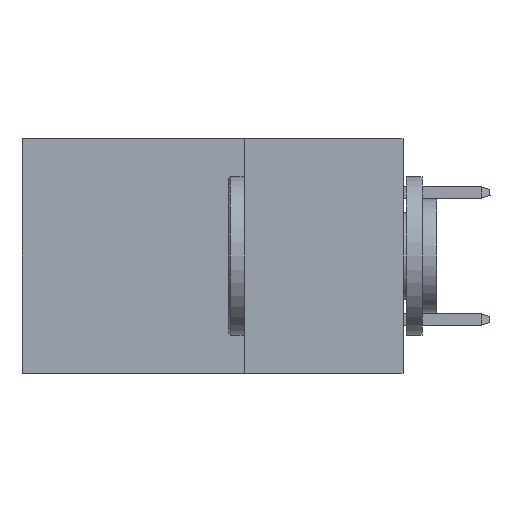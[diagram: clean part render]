
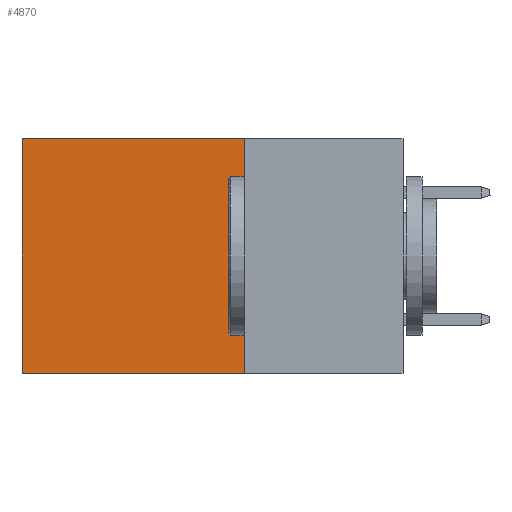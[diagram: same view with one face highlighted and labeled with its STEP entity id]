
A CAD part, left-side view. The second image highlights one B-rep face of the part: STEP entity #4870.
In plain terms, the highlighted planar face has unit normal (-1, 0, 0).
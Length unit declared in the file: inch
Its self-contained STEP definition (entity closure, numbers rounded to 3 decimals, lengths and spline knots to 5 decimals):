
#151 = AXIS2_PLACEMENT_3D ( 'NONE', #30041, #43846, #37055 ) ;
#203 = EDGE_CURVE ( 'NONE', #12545, #15745, #37121, .T. ) ;
#1642 = CARTESIAN_POINT ( 'NONE',  ( 0.2875, 0.25, 0. ) ) ;
#4870 = ADVANCED_FACE ( 'NONE', ( #23007 ), #40685, .F. ) ;
#5103 = ORIENTED_EDGE ( 'NONE', *, *, #34790, .T. ) ;
#6206 = VERTEX_POINT ( 'NONE', #18463 ) ;
#10117 = DIRECTION ( 'NONE',  ( 0., 1., 0. ) ) ;
#12295 = LINE ( 'NONE', #39982, #25549 ) ;
#12545 = VERTEX_POINT ( 'NONE', #40342 ) ;
#14321 = CARTESIAN_POINT ( 'NONE',  ( 0.2875, 0.25, 0. ) ) ;
#14422 = CARTESIAN_POINT ( 'NONE',  ( 0.2875, 0.6, 0. ) ) ;
#15745 = VERTEX_POINT ( 'NONE', #18580 ) ;
#18463 = CARTESIAN_POINT ( 'NONE',  ( 0.2875, 0.25, 0. ) ) ;
#18580 = CARTESIAN_POINT ( 'NONE',  ( 0.2875, 0.6, -0.37 ) ) ;
#19726 = EDGE_CURVE ( 'NONE', #26175, #15745, #12295, .T. ) ;
#21597 = DIRECTION ( 'NONE',  ( 0., 1., 0. ) ) ;
#23007 = FACE_OUTER_BOUND ( 'NONE', #35587, .T. ) ;
#25208 = LINE ( 'NONE', #14321, #28361 ) ;
#25549 = VECTOR ( 'NONE', #26623, 39.37008 ) ;
#26175 = VERTEX_POINT ( 'NONE', #14422 ) ;
#26623 = DIRECTION ( 'NONE',  ( 0., 0., -1. ) ) ;
#28361 = VECTOR ( 'NONE', #39010, 39.37008 ) ;
#28862 = LINE ( 'NONE', #1642, #35869 ) ;
#29438 = ORIENTED_EDGE ( 'NONE', *, *, #203, .F. ) ;
#30041 = CARTESIAN_POINT ( 'NONE',  ( 0.2875, 0.25, 0. ) ) ;
#33960 = ORIENTED_EDGE ( 'NONE', *, *, #19726, .T. ) ;
#34790 = EDGE_CURVE ( 'NONE', #6206, #26175, #28862, .T. ) ;
#35587 = EDGE_LOOP ( 'NONE', ( #33960, #29438, #43714, #5103 ) ) ;
#35869 = VECTOR ( 'NONE', #21597, 39.37008 ) ;
#37055 = DIRECTION ( 'NONE',  ( 0., 0., -1. ) ) ;
#37121 = LINE ( 'NONE', #40967, #40025 ) ;
#39010 = DIRECTION ( 'NONE',  ( 0., 0., -1. ) ) ;
#39982 = CARTESIAN_POINT ( 'NONE',  ( 0.2875, 0.6, 0. ) ) ;
#40025 = VECTOR ( 'NONE', #10117, 39.37008 ) ;
#40342 = CARTESIAN_POINT ( 'NONE',  ( 0.2875, 0.25, -0.37 ) ) ;
#40685 = PLANE ( 'NONE',  #151 ) ;
#40967 = CARTESIAN_POINT ( 'NONE',  ( 0.2875, 0.25, -0.37 ) ) ;
#43496 = EDGE_CURVE ( 'NONE', #6206, #12545, #25208, .T. ) ;
#43714 = ORIENTED_EDGE ( 'NONE', *, *, #43496, .F. ) ;
#43846 = DIRECTION ( 'NONE',  ( 1., 0., 0. ) ) ;
